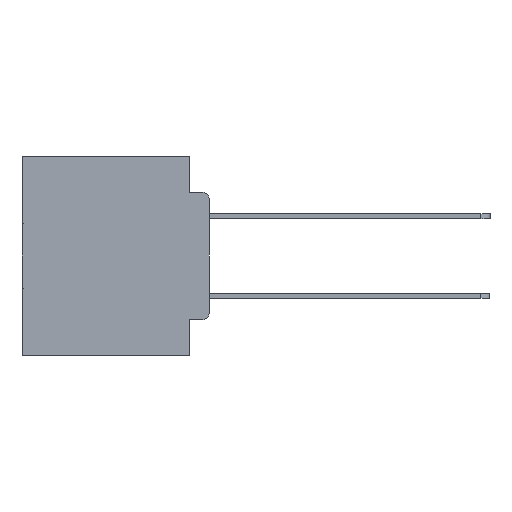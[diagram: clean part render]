
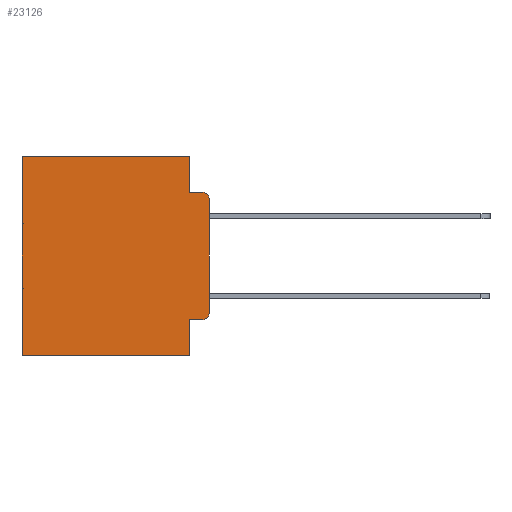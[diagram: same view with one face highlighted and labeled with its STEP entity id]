
A CAD part, left-side view. The second image highlights one B-rep face of the part: STEP entity #23126.
In plain terms, the highlighted planar face has unit normal (-1, 0, 0).
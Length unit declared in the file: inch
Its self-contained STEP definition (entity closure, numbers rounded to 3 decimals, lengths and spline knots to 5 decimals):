
#115 = VERTEX_POINT ( 'NONE', #22154 ) ;
#385 = EDGE_CURVE ( 'NONE', #115, #13471, #28788, .T. ) ;
#453 = CARTESIAN_POINT ( 'NONE',  ( 0.298, 0.02, -0.4115 ) ) ;
#498 = VECTOR ( 'NONE', #17845, 39.37008 ) ;
#1467 = EDGE_CURVE ( 'NONE', #10157, #7683, #31831, .T. ) ;
#2413 = ORIENTED_EDGE ( 'NONE', *, *, #22263, .T. ) ;
#2587 = CARTESIAN_POINT ( 'NONE',  ( 0.298, 0.051, -0.5 ) ) ;
#3161 = VECTOR ( 'NONE', #11691, 39.37008 ) ;
#3296 = CIRCLE ( 'NONE', #19596, 0.02 ) ;
#3316 = DIRECTION ( 'NONE',  ( 0., 0., -1. ) ) ;
#3704 = LINE ( 'NONE', #23359, #4490 ) ;
#4490 = VECTOR ( 'NONE', #5458, 39.37008 ) ;
#4787 = DIRECTION ( 'NONE',  ( -1., 0., 0. ) ) ;
#5126 = EDGE_CURVE ( 'NONE', #13471, #6359, #23332, .T. ) ;
#5299 = CARTESIAN_POINT ( 'NONE',  ( 0.298, 0.02, -0.0885 ) ) ;
#5458 = DIRECTION ( 'NONE',  ( 0., 0., -1. ) ) ;
#5573 = CARTESIAN_POINT ( 'NONE',  ( 0.298, 0.051, -0.0885 ) ) ;
#6112 = VERTEX_POINT ( 'NONE', #17884 ) ;
#6359 = VERTEX_POINT ( 'NONE', #5299 ) ;
#7515 = CARTESIAN_POINT ( 'NONE',  ( 0.298, 0.051, -0.4115 ) ) ;
#7561 = ORIENTED_EDGE ( 'NONE', *, *, #32184, .T. ) ;
#7683 = VERTEX_POINT ( 'NONE', #2587 ) ;
#8061 = PLANE ( 'NONE',  #20797 ) ;
#8361 = CARTESIAN_POINT ( 'NONE',  ( 0.298, 0.02, -0.3915 ) ) ;
#9147 = ORIENTED_EDGE ( 'NONE', *, *, #24363, .F. ) ;
#9737 = EDGE_CURVE ( 'NONE', #7683, #6112, #10754, .T. ) ;
#9955 = CARTESIAN_POINT ( 'NONE',  ( 0.298, 0.473, 0. ) ) ;
#10120 = DIRECTION ( 'NONE',  ( 0., -1., 0. ) ) ;
#10157 = VERTEX_POINT ( 'NONE', #28381 ) ;
#10691 = DIRECTION ( 'NONE',  ( 0., 0., -1. ) ) ;
#10754 = LINE ( 'NONE', #29372, #3161 ) ;
#10995 = VECTOR ( 'NONE', #10120, 39.37008 ) ;
#11005 = DIRECTION ( 'NONE',  ( 0., 0., -1. ) ) ;
#11529 = VERTEX_POINT ( 'NONE', #453 ) ;
#11691 = DIRECTION ( 'NONE',  ( 0., 1., 0. ) ) ;
#12416 = ORIENTED_EDGE ( 'NONE', *, *, #5126, .F. ) ;
#12603 = FACE_OUTER_BOUND ( 'NONE', #31662, .T. ) ;
#12845 = VECTOR ( 'NONE', #13275, 39.37008 ) ;
#13275 = DIRECTION ( 'NONE',  ( 0., 1., 0. ) ) ;
#13471 = VERTEX_POINT ( 'NONE', #5573 ) ;
#13482 = VERTEX_POINT ( 'NONE', #15824 ) ;
#13630 = CARTESIAN_POINT ( 'NONE',  ( 0.298, 0.051, 0. ) ) ;
#13645 = LINE ( 'NONE', #28403, #12845 ) ;
#14141 = EDGE_CURVE ( 'NONE', #23862, #6112, #20931, .T. ) ;
#14684 = EDGE_CURVE ( 'NONE', #13482, #6359, #3296, .T. ) ;
#15824 = CARTESIAN_POINT ( 'NONE',  ( 0.298, 0., -0.1085 ) ) ;
#16479 = ORIENTED_EDGE ( 'NONE', *, *, #25568, .T. ) ;
#16600 = VECTOR ( 'NONE', #25481, 39.37008 ) ;
#17041 = LINE ( 'NONE', #7515, #10995 ) ;
#17845 = DIRECTION ( 'NONE',  ( 0., 0., -1. ) ) ;
#17884 = CARTESIAN_POINT ( 'NONE',  ( 0.298, 0.473, -0.5 ) ) ;
#19040 = CIRCLE ( 'NONE', #29356, 0.02 ) ;
#19596 = AXIS2_PLACEMENT_3D ( 'NONE', #20125, #4787, #22703 ) ;
#19645 = ORIENTED_EDGE ( 'NONE', *, *, #1467, .F. ) ;
#20125 = CARTESIAN_POINT ( 'NONE',  ( 0.298, 0.02, -0.1085 ) ) ;
#20780 = CARTESIAN_POINT ( 'NONE',  ( 0.298, 0., 0. ) ) ;
#20797 = AXIS2_PLACEMENT_3D ( 'NONE', #20780, #25937, #10691 ) ;
#20831 = ORIENTED_EDGE ( 'NONE', *, *, #385, .F. ) ;
#20931 = LINE ( 'NONE', #9955, #498 ) ;
#22154 = CARTESIAN_POINT ( 'NONE',  ( 0.298, 0.051, 0. ) ) ;
#22263 = EDGE_CURVE ( 'NONE', #11529, #31728, #19040, .T. ) ;
#22703 = DIRECTION ( 'NONE',  ( 0., 0., -1. ) ) ;
#23126 = ADVANCED_FACE ( 'NONE', ( #12603 ), #8061, .F. ) ;
#23332 = LINE ( 'NONE', #30347, #16600 ) ;
#23359 = CARTESIAN_POINT ( 'NONE',  ( 0.298, 0., 0. ) ) ;
#23862 = VERTEX_POINT ( 'NONE', #23938 ) ;
#23938 = CARTESIAN_POINT ( 'NONE',  ( 0.298, 0.473, 0. ) ) ;
#24363 = EDGE_CURVE ( 'NONE', #13482, #31728, #3704, .T. ) ;
#24386 = ORIENTED_EDGE ( 'NONE', *, *, #14684, .T. ) ;
#24775 = ORIENTED_EDGE ( 'NONE', *, *, #9737, .F. ) ;
#25481 = DIRECTION ( 'NONE',  ( 0., -1., 0. ) ) ;
#25520 = CARTESIAN_POINT ( 'NONE',  ( 0.298, 0.051, 0. ) ) ;
#25568 = EDGE_CURVE ( 'NONE', #115, #23862, #13645, .T. ) ;
#25937 = DIRECTION ( 'NONE',  ( 1., 0., 0. ) ) ;
#25985 = CARTESIAN_POINT ( 'NONE',  ( 0.298, 0., -0.3915 ) ) ;
#26239 = DIRECTION ( 'NONE',  ( -1., 0., 0. ) ) ;
#28012 = VECTOR ( 'NONE', #3316, 39.37008 ) ;
#28381 = CARTESIAN_POINT ( 'NONE',  ( 0.298, 0.051, -0.4115 ) ) ;
#28403 = CARTESIAN_POINT ( 'NONE',  ( 0.298, 0., 0. ) ) ;
#28788 = LINE ( 'NONE', #13630, #28012 ) ;
#29356 = AXIS2_PLACEMENT_3D ( 'NONE', #8361, #26239, #11005 ) ;
#29372 = CARTESIAN_POINT ( 'NONE',  ( 0.298, 0., -0.5 ) ) ;
#29805 = ORIENTED_EDGE ( 'NONE', *, *, #14141, .T. ) ;
#30302 = VECTOR ( 'NONE', #31156, 39.37008 ) ;
#30347 = CARTESIAN_POINT ( 'NONE',  ( 0.298, 0.051, -0.0885 ) ) ;
#31156 = DIRECTION ( 'NONE',  ( 0., 0., -1. ) ) ;
#31662 = EDGE_LOOP ( 'NONE', ( #9147, #24386, #12416, #20831, #16479, #29805, #24775, #19645, #7561, #2413 ) ) ;
#31728 = VERTEX_POINT ( 'NONE', #25985 ) ;
#31831 = LINE ( 'NONE', #25520, #30302 ) ;
#32184 = EDGE_CURVE ( 'NONE', #10157, #11529, #17041, .T. ) ;
